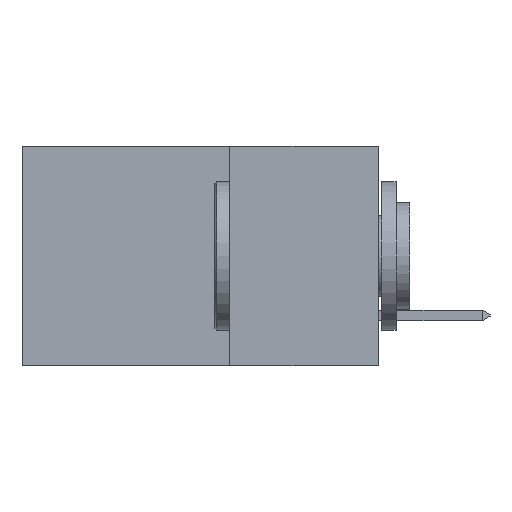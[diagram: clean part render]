
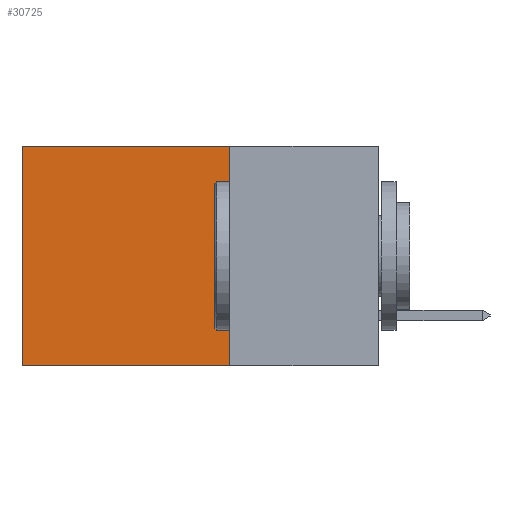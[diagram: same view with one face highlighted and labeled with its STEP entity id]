
A CAD part, left-side view. The second image highlights one B-rep face of the part: STEP entity #30725.
In plain terms, the highlighted planar face has unit normal (-1, 0, 0).
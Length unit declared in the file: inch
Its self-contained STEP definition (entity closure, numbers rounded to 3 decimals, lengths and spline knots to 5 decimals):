
#35 = EDGE_CURVE ( 'NONE', #2536, #21790, #8154, .T. ) ;
#132 = CARTESIAN_POINT ( 'NONE',  ( 0.298, 0.6, -0.37 ) ) ;
#2536 = VERTEX_POINT ( 'NONE', #31807 ) ;
#4876 = EDGE_CURVE ( 'NONE', #21790, #19593, #31231, .T. ) ;
#5612 = CARTESIAN_POINT ( 'NONE',  ( 0.298, 0.6, 0. ) ) ;
#8154 = LINE ( 'NONE', #16910, #21416 ) ;
#9236 = ORIENTED_EDGE ( 'NONE', *, *, #35, .T. ) ;
#9778 = ORIENTED_EDGE ( 'NONE', *, *, #26301, .F. ) ;
#10004 = FACE_OUTER_BOUND ( 'NONE', #28835, .T. ) ;
#10702 = LINE ( 'NONE', #27357, #23189 ) ;
#11538 = AXIS2_PLACEMENT_3D ( 'NONE', #30901, #25960, #26072 ) ;
#12008 = DIRECTION ( 'NONE',  ( 0., 0., -1. ) ) ;
#12399 = DIRECTION ( 'NONE',  ( 0., 1., 0. ) ) ;
#13941 = VECTOR ( 'NONE', #25584, 39.37008 ) ;
#15823 = ORIENTED_EDGE ( 'NONE', *, *, #22473, .F. ) ;
#16910 = CARTESIAN_POINT ( 'NONE',  ( 0.298, 0.25, 0. ) ) ;
#17279 = VECTOR ( 'NONE', #12008, 39.37008 ) ;
#19567 = CARTESIAN_POINT ( 'NONE',  ( 0.298, 0.25, -0.37 ) ) ;
#19593 = VERTEX_POINT ( 'NONE', #132 ) ;
#20244 = DIRECTION ( 'NONE',  ( 0., 1., 0. ) ) ;
#20606 = ORIENTED_EDGE ( 'NONE', *, *, #4876, .T. ) ;
#21059 = PLANE ( 'NONE',  #11538 ) ;
#21416 = VECTOR ( 'NONE', #20244, 39.37008 ) ;
#21790 = VERTEX_POINT ( 'NONE', #5612 ) ;
#22473 = EDGE_CURVE ( 'NONE', #2536, #29478, #27226, .T. ) ;
#22898 = CARTESIAN_POINT ( 'NONE',  ( 0.298, 0.6, 0. ) ) ;
#23042 = CARTESIAN_POINT ( 'NONE',  ( 0.298, 0.25, 0. ) ) ;
#23189 = VECTOR ( 'NONE', #12399, 39.37008 ) ;
#25584 = DIRECTION ( 'NONE',  ( 0., 0., -1. ) ) ;
#25960 = DIRECTION ( 'NONE',  ( 1., 0., 0. ) ) ;
#26072 = DIRECTION ( 'NONE',  ( 0., 0., -1. ) ) ;
#26301 = EDGE_CURVE ( 'NONE', #29478, #19593, #10702, .T. ) ;
#27226 = LINE ( 'NONE', #23042, #13941 ) ;
#27357 = CARTESIAN_POINT ( 'NONE',  ( 0.298, 0.25, -0.37 ) ) ;
#28835 = EDGE_LOOP ( 'NONE', ( #20606, #9778, #15823, #9236 ) ) ;
#29478 = VERTEX_POINT ( 'NONE', #19567 ) ;
#30725 = ADVANCED_FACE ( 'NONE', ( #10004 ), #21059, .F. ) ;
#30901 = CARTESIAN_POINT ( 'NONE',  ( 0.298, 0.25, 0. ) ) ;
#31231 = LINE ( 'NONE', #22898, #17279 ) ;
#31807 = CARTESIAN_POINT ( 'NONE',  ( 0.298, 0.25, 0. ) ) ;
